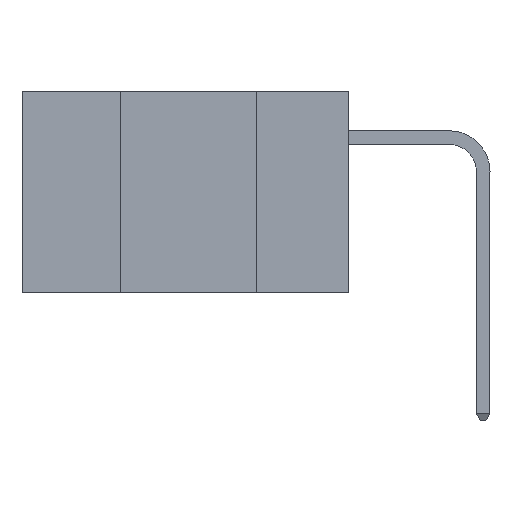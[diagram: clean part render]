
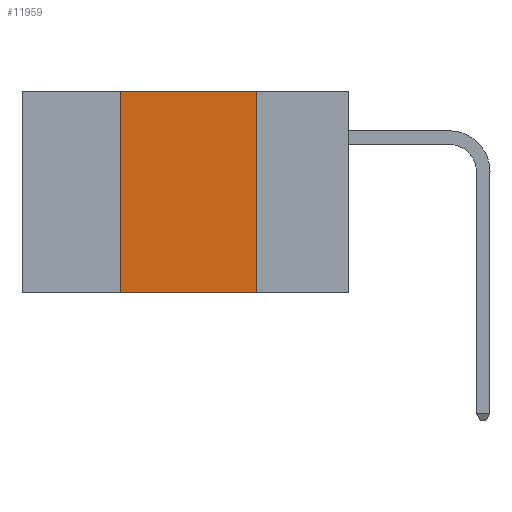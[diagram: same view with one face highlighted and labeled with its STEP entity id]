
A CAD part, left-side view. The second image highlights one B-rep face of the part: STEP entity #11959.
In plain terms, the highlighted planar face has unit normal (-1, 0, 0).
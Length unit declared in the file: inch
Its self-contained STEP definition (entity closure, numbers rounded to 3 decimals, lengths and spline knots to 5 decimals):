
#148 = VERTEX_POINT ( 'NONE', #12938 ) ;
#1731 = EDGE_CURVE ( 'NONE', #148, #10339, #12068, .T. ) ;
#2179 = DIRECTION ( 'NONE',  ( 0., 0., -1. ) ) ;
#2945 = LINE ( 'NONE', #28685, #14409 ) ;
#4505 = CARTESIAN_POINT ( 'NONE',  ( 0., 0.17, -0.37 ) ) ;
#4573 = DIRECTION ( 'NONE',  ( 0., -1., 0. ) ) ;
#6224 = EDGE_CURVE ( 'NONE', #30995, #10339, #36565, .T. ) ;
#7707 = CARTESIAN_POINT ( 'NONE',  ( 0., 0.17, 0. ) ) ;
#8696 = EDGE_CURVE ( 'NONE', #30995, #19317, #2945, .T. ) ;
#8864 = CARTESIAN_POINT ( 'NONE',  ( 0., 0.42, -0.37 ) ) ;
#9641 = LINE ( 'NONE', #21700, #10514 ) ;
#10339 = VERTEX_POINT ( 'NONE', #4505 ) ;
#10514 = VECTOR ( 'NONE', #24601, 39.37008 ) ;
#11184 = DIRECTION ( 'NONE',  ( 0., 0., 1. ) ) ;
#11959 = ADVANCED_FACE ( 'NONE', ( #26014 ), #29575, .F. ) ;
#12068 = LINE ( 'NONE', #7707, #25282 ) ;
#12088 = CARTESIAN_POINT ( 'NONE',  ( 0., 0.6, 0. ) ) ;
#12938 = CARTESIAN_POINT ( 'NONE',  ( 0., 0.17, 0. ) ) ;
#13109 = ORIENTED_EDGE ( 'NONE', *, *, #6224, .T. ) ;
#14409 = VECTOR ( 'NONE', #11184, 39.37008 ) ;
#19317 = VERTEX_POINT ( 'NONE', #37493 ) ;
#21700 = CARTESIAN_POINT ( 'NONE',  ( 0., 0.6, 0. ) ) ;
#22183 = CARTESIAN_POINT ( 'NONE',  ( 0., 0.6, -0.37 ) ) ;
#22867 = ORIENTED_EDGE ( 'NONE', *, *, #8696, .F. ) ;
#23801 = DIRECTION ( 'NONE',  ( 0., 0., -1. ) ) ;
#24601 = DIRECTION ( 'NONE',  ( 0., -1., 0. ) ) ;
#25282 = VECTOR ( 'NONE', #2179, 39.37008 ) ;
#26014 = FACE_OUTER_BOUND ( 'NONE', #30375, .T. ) ;
#28518 = EDGE_CURVE ( 'NONE', #19317, #148, #9641, .T. ) ;
#28685 = CARTESIAN_POINT ( 'NONE',  ( 0., 0.42, 0. ) ) ;
#29575 = PLANE ( 'NONE',  #34896 ) ;
#29955 = DIRECTION ( 'NONE',  ( 1., 0., 0. ) ) ;
#30375 = EDGE_LOOP ( 'NONE', ( #31027, #30869, #22867, #13109 ) ) ;
#30869 = ORIENTED_EDGE ( 'NONE', *, *, #28518, .F. ) ;
#30995 = VERTEX_POINT ( 'NONE', #8864 ) ;
#31027 = ORIENTED_EDGE ( 'NONE', *, *, #1731, .F. ) ;
#34896 = AXIS2_PLACEMENT_3D ( 'NONE', #12088, #29955, #23801 ) ;
#36127 = VECTOR ( 'NONE', #4573, 39.37008 ) ;
#36565 = LINE ( 'NONE', #22183, #36127 ) ;
#37493 = CARTESIAN_POINT ( 'NONE',  ( 0., 0.42, 0. ) ) ;
